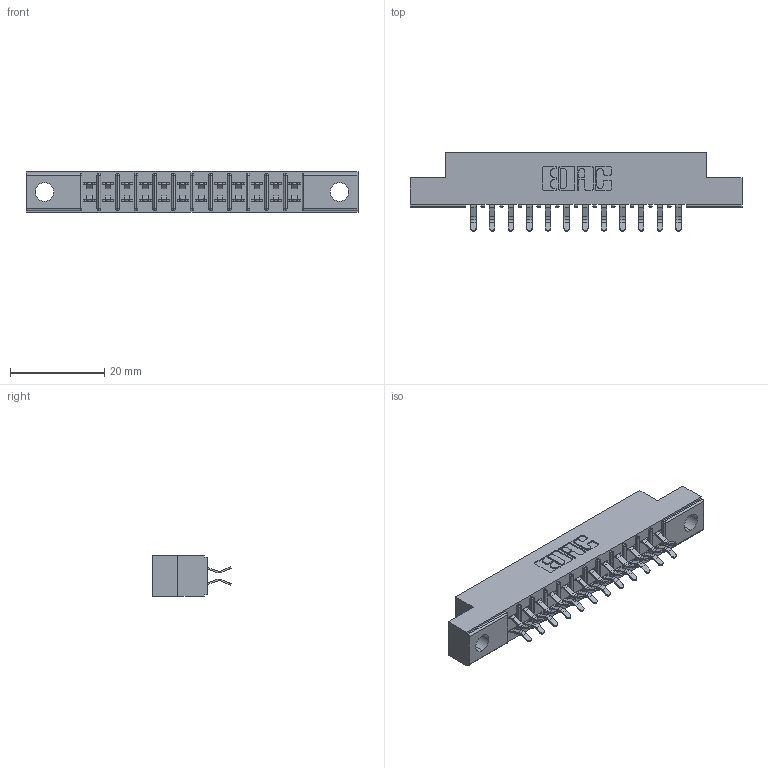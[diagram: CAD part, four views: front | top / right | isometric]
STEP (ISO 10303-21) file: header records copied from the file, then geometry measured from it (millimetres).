
FILE_DESCRIPTION (( 'STEP AP203' ), '1' );
FILE_NAME ('355-024-556-204.STEP', '2019-09-11T05:06:04', ( '' ), ( '' ), 'SwSTEP 2.0', 'SolidWorks 2016', '' );
FILE_SCHEMA (( 'CONFIG_CONTROL_DESIGN' ));
Length unit declared in the file: inch
Products named in the file (3): 305 Part_.156 Dia; 305-290-001_556; 355-024-556-204
Assembly tree (25 placements, depth 2):
  355-024-556-204
    305 Part_.156 Dia
    305-290-001_556  x24
Bounding box: 70.56 x 16.64 x 8.71 mm (x, y, z)
Volume: 4327.1 mm3; surface area: 7504.4 mm2
Topology: 25 solids, 25 shells, 1474 faces, 4228 edges, 2752 vertices
Faces by surface type: plane 826, cylinder 600, sphere 48
Entity records: 17285 total; most frequent: CARTESIAN_POINT 2868, ORIENTED_EDGE 2840, DIRECTION 2794, EDGE_CURVE 1420, VECTOR 1118, LINE 1118, VERTEX_POINT 912, AXIS2_PLACEMENT_3D 838
